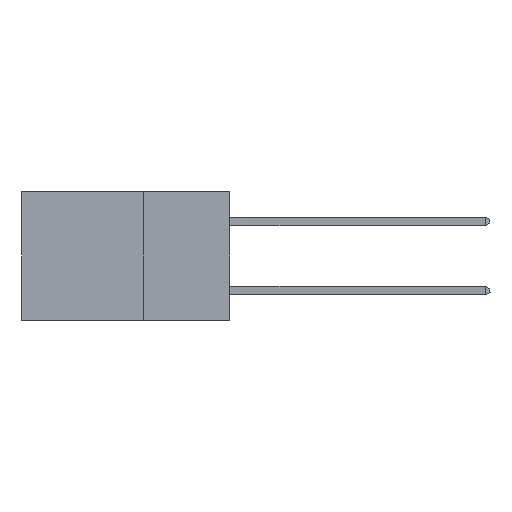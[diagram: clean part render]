
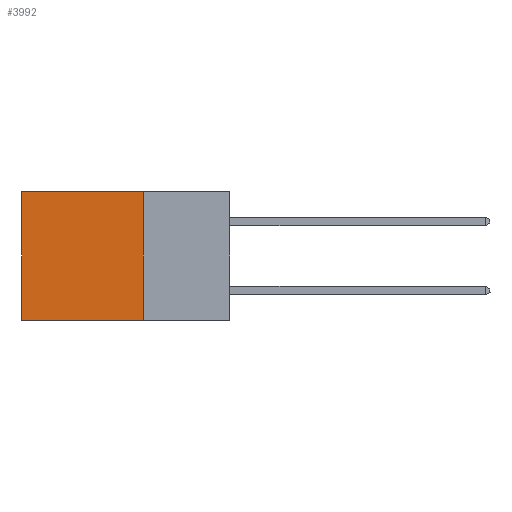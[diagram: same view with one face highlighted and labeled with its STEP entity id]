
A CAD part, left-side view. The second image highlights one B-rep face of the part: STEP entity #3992.
In plain terms, the highlighted planar face has unit normal (-1, 0, 0).
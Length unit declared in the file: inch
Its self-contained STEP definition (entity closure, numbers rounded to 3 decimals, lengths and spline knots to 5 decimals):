
#217 = EDGE_CURVE ( 'NONE', #1465, #6074, #6432, .T. ) ;
#256 = CARTESIAN_POINT ( 'NONE',  ( 0.298, 0.6, 0. ) ) ;
#1295 = DIRECTION ( 'NONE',  ( 0., 1., 0. ) ) ;
#1465 = VERTEX_POINT ( 'NONE', #3264 ) ;
#2409 = CARTESIAN_POINT ( 'NONE',  ( 0.298, 0.25, -0.37 ) ) ;
#2515 = VECTOR ( 'NONE', #5921, 39.37008 ) ;
#2548 = FACE_OUTER_BOUND ( 'NONE', #10807, .T. ) ;
#2578 = ORIENTED_EDGE ( 'NONE', *, *, #9525, .T. ) ;
#3051 = DIRECTION ( 'NONE',  ( 0., 0., -1. ) ) ;
#3264 = CARTESIAN_POINT ( 'NONE',  ( 0.298, 0.25, 0. ) ) ;
#3992 = ADVANCED_FACE ( 'NONE', ( #2548 ), #5969, .F. ) ;
#4415 = CARTESIAN_POINT ( 'NONE',  ( 0.298, 0.25, -0.37 ) ) ;
#5077 = LINE ( 'NONE', #2409, #6795 ) ;
#5314 = EDGE_CURVE ( 'NONE', #1465, #9858, #5593, .T. ) ;
#5593 = LINE ( 'NONE', #6879, #7515 ) ;
#5770 = AXIS2_PLACEMENT_3D ( 'NONE', #9317, #8361, #3051 ) ;
#5921 = DIRECTION ( 'NONE',  ( 0., 0., -1. ) ) ;
#5969 = PLANE ( 'NONE',  #5770 ) ;
#6074 = VERTEX_POINT ( 'NONE', #8405 ) ;
#6405 = VERTEX_POINT ( 'NONE', #12216 ) ;
#6432 = LINE ( 'NONE', #8810, #8819 ) ;
#6795 = VECTOR ( 'NONE', #1295, 39.37008 ) ;
#6879 = CARTESIAN_POINT ( 'NONE',  ( 0.298, 0.25, 0. ) ) ;
#7515 = VECTOR ( 'NONE', #11040, 39.37008 ) ;
#8361 = DIRECTION ( 'NONE',  ( 1., 0., 0. ) ) ;
#8405 = CARTESIAN_POINT ( 'NONE',  ( 0.298, 0.6, 0. ) ) ;
#8552 = ORIENTED_EDGE ( 'NONE', *, *, #217, .T. ) ;
#8810 = CARTESIAN_POINT ( 'NONE',  ( 0.298, 0.25, 0. ) ) ;
#8819 = VECTOR ( 'NONE', #13853, 39.37008 ) ;
#9317 = CARTESIAN_POINT ( 'NONE',  ( 0.298, 0.25, 0. ) ) ;
#9525 = EDGE_CURVE ( 'NONE', #6074, #6405, #12832, .T. ) ;
#9777 = ORIENTED_EDGE ( 'NONE', *, *, #5314, .F. ) ;
#9858 = VERTEX_POINT ( 'NONE', #4415 ) ;
#10355 = EDGE_CURVE ( 'NONE', #9858, #6405, #5077, .T. ) ;
#10807 = EDGE_LOOP ( 'NONE', ( #2578, #13393, #9777, #8552 ) ) ;
#11040 = DIRECTION ( 'NONE',  ( 0., 0., -1. ) ) ;
#12216 = CARTESIAN_POINT ( 'NONE',  ( 0.298, 0.6, -0.37 ) ) ;
#12832 = LINE ( 'NONE', #256, #2515 ) ;
#13393 = ORIENTED_EDGE ( 'NONE', *, *, #10355, .F. ) ;
#13853 = DIRECTION ( 'NONE',  ( 0., 1., 0. ) ) ;
